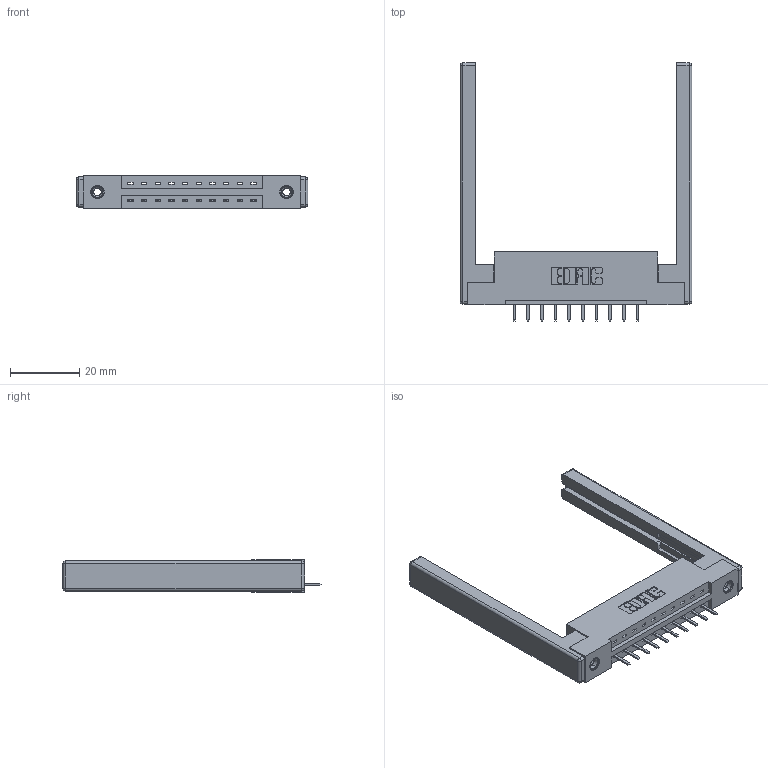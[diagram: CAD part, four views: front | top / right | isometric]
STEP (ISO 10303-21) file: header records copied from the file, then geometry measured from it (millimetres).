
FILE_DESCRIPTION (( 'STEP AP203' ), '1' );
FILE_NAME ('337-010-520-168.STEP', '2019-09-27T20:58:11', ( '' ), ( '' ), 'SwSTEP 2.0', 'SolidWorks 2016', '' );
FILE_SCHEMA (( 'CONFIG_CONTROL_DESIGN' ));
Length unit declared in the file: inch
Products named in the file (5): 345-250-001_345-250-001-102; 345-292-001_345-293-120; 337-010-520-168; 307-220-068; 337 Part_Flush Mounting Lugs - 0.156 Dia-TI
Assembly tree (15 placements, depth 2):
  337-010-520-168
    337 Part_Flush Mounting Lugs - 0.156 Dia-TI
    345-292-001_345-293-120  x10
    345-250-001_345-250-001-102  x2
    307-220-068  x2
Bounding box: 67.06 x 74.76 x 9.4 mm (x, y, z)
Volume: 10931.4 mm3; surface area: 10569.8 mm2
Topology: 15 solids, 15 shells, 928 faces, 2661 edges, 1726 vertices
Faces by surface type: plane 638, cylinder 266, cone 12, sphere 8, torus 4
Entity records: 14446 total; most frequent: CARTESIAN_POINT 2481, ORIENTED_EDGE 2404, DIRECTION 2216, EDGE_CURVE 1202, VECTOR 1020, LINE 1020, VERTEX_POINT 790, AXIS2_PLACEMENT_3D 598
